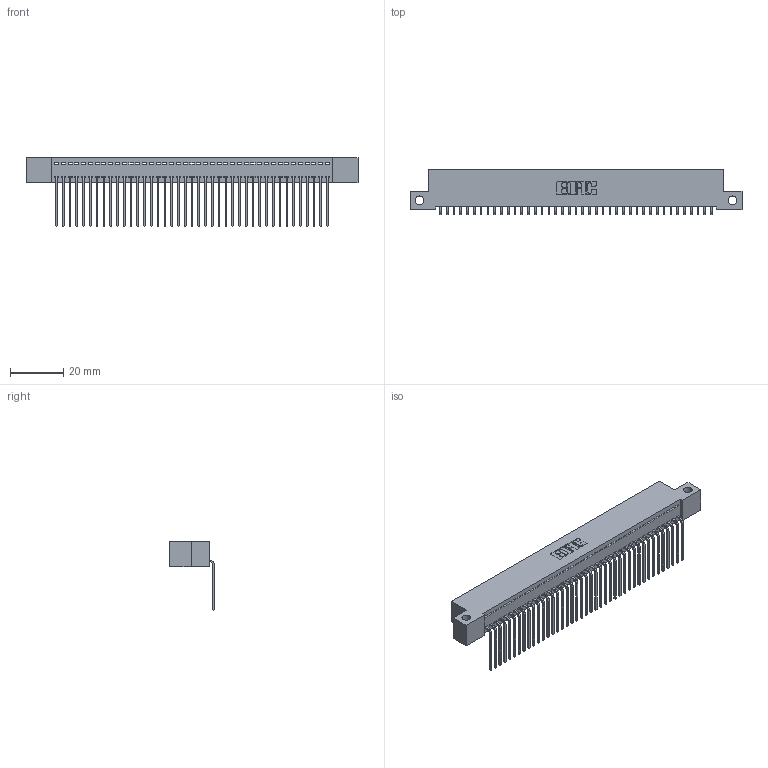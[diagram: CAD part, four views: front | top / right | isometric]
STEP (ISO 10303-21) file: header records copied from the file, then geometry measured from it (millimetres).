
FILE_DESCRIPTION (( 'STEP AP203' ), '1' );
FILE_NAME ('342-041-559-112.STEP', '2018-08-12T02:02:47', ( '' ), ( '' ), 'SwSTEP 2.0', 'SolidWorks 2016', '' );
FILE_SCHEMA (( 'CONFIG_CONTROL_DESIGN' ));
Length unit declared in the file: inch
Products named in the file (3): 342 Part_Side Mount; 345-292-001_558 559 Tail - 1; 342-041-559-112
Assembly tree (42 placements, depth 2):
  342-041-559-112
    342 Part_Side Mount
    345-292-001_558 559 Tail - 1  x41
Bounding box: 124.46 x 16.83 x 25.78 mm (x, y, z)
Volume: 10971.6 mm3; surface area: 16705.4 mm2
Topology: 42 solids, 42 shells, 2570 faces, 7761 edges, 5118 vertices
Faces by surface type: plane 1870, cylinder 700
Entity records: 25149 total; most frequent: CARTESIAN_POINT 4345, ORIENTED_EDGE 4322, DIRECTION 3667, EDGE_CURVE 2161, LINE 2033, VECTOR 2033, VERTEX_POINT 1438, AXIS2_PLACEMENT_3D 817
